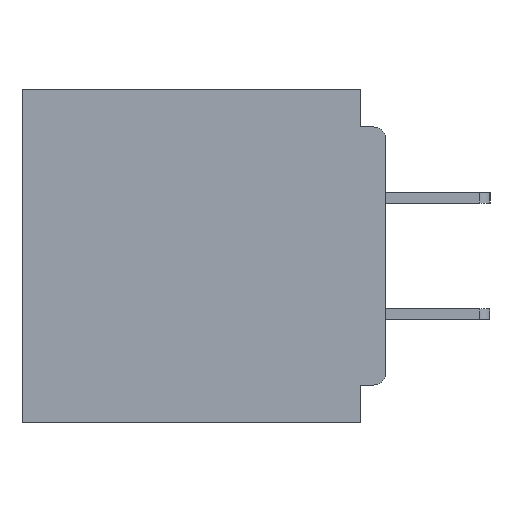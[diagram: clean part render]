
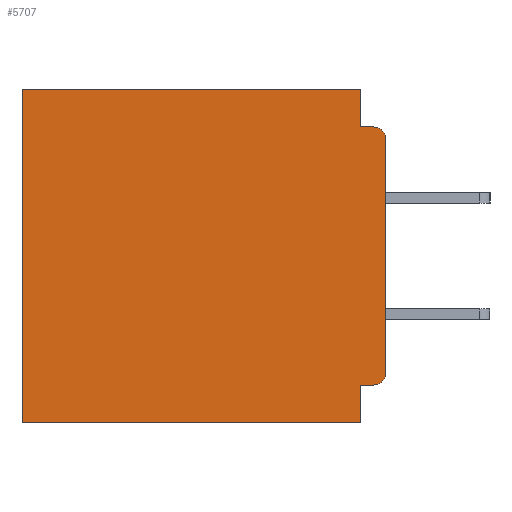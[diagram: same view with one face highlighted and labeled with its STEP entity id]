
A CAD part, left-side view. The second image highlights one B-rep face of the part: STEP entity #5707.
In plain terms, the highlighted planar face has unit normal (-1, 0, 0).
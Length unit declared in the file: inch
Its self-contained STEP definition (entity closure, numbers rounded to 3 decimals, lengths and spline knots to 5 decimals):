
#2640 = CARTESIAN_POINT ( 'NONE',  ( 0.3, 0.031, -0.045 ) ) ;
#3338 = CARTESIAN_POINT ( 'NONE',  ( 0.3, 0.031, -0.355 ) ) ;
#3873 = VECTOR ( 'NONE', #16512, 39.37008 ) ;
#4397 = EDGE_CURVE ( 'NONE', #32176, #6523, #39195, .T. ) ;
#4550 = EDGE_CURVE ( 'NONE', #6523, #17358, #5395, .T. ) ;
#4761 = CARTESIAN_POINT ( 'NONE',  ( 0.3, 0., -0.06 ) ) ;
#4972 = EDGE_LOOP ( 'NONE', ( #5251, #22607, #36116, #38105, #28368, #12753, #35700, #60709, #61711, #25849 ) ) ;
#5251 = ORIENTED_EDGE ( 'NONE', *, *, #47994, .F. ) ;
#5395 = LINE ( 'NONE', #31305, #3873 ) ;
#5631 = CIRCLE ( 'NONE', #12392, 0.015 ) ;
#5706 = EDGE_CURVE ( 'NONE', #32176, #54962, #39880, .T. ) ;
#5707 = ADVANCED_FACE ( 'NONE', ( #54378 ), #25562, .F. ) ;
#6001 = DIRECTION ( 'NONE',  ( -1., 0., 0. ) ) ;
#6523 = VERTEX_POINT ( 'NONE', #3338 ) ;
#7108 = LINE ( 'NONE', #30990, #31738 ) ;
#8155 = CARTESIAN_POINT ( 'NONE',  ( 0.3, 0., -0.34 ) ) ;
#8298 = CARTESIAN_POINT ( 'NONE',  ( 0.3, 0.437, -0.4 ) ) ;
#8431 = LINE ( 'NONE', #8298, #19957 ) ;
#9497 = CARTESIAN_POINT ( 'NONE',  ( 0.3, 0., -0.4 ) ) ;
#10766 = CARTESIAN_POINT ( 'NONE',  ( 0.3, 0.015, -0.355 ) ) ;
#10851 = VECTOR ( 'NONE', #26500, 39.37008 ) ;
#10919 = DIRECTION ( 'NONE',  ( 1., 0., 0. ) ) ;
#11439 = AXIS2_PLACEMENT_3D ( 'NONE', #35404, #6001, #40308 ) ;
#12392 = AXIS2_PLACEMENT_3D ( 'NONE', #43758, #14448, #48666 ) ;
#12753 = ORIENTED_EDGE ( 'NONE', *, *, #14471, .T. ) ;
#13203 = CARTESIAN_POINT ( 'NONE',  ( 0.3, 0., 0. ) ) ;
#13997 = CARTESIAN_POINT ( 'NONE',  ( 0.3, 0.437, -0.4 ) ) ;
#14448 = DIRECTION ( 'NONE',  ( -1., 0., 0. ) ) ;
#14471 = EDGE_CURVE ( 'NONE', #35315, #16813, #8431, .T. ) ;
#15427 = DIRECTION ( 'NONE',  ( 0., 1., 0. ) ) ;
#16512 = DIRECTION ( 'NONE',  ( 0., 0., -1. ) ) ;
#16813 = VERTEX_POINT ( 'NONE', #13997 ) ;
#17358 = VERTEX_POINT ( 'NONE', #57992 ) ;
#18377 = CARTESIAN_POINT ( 'NONE',  ( 0.3, 0., -0.4 ) ) ;
#19957 = VECTOR ( 'NONE', #37678, 39.37008 ) ;
#20743 = CARTESIAN_POINT ( 'NONE',  ( 0.3, 0.015, -0.045 ) ) ;
#22418 = LINE ( 'NONE', #55731, #10851 ) ;
#22607 = ORIENTED_EDGE ( 'NONE', *, *, #32516, .T. ) ;
#23160 = VECTOR ( 'NONE', #57064, 39.37008 ) ;
#24619 = AXIS2_PLACEMENT_3D ( 'NONE', #40106, #10919, #45216 ) ;
#25562 = PLANE ( 'NONE',  #24619 ) ;
#25849 = ORIENTED_EDGE ( 'NONE', *, *, #5706, .T. ) ;
#26191 = VECTOR ( 'NONE', #15427, 39.37008 ) ;
#26319 = EDGE_CURVE ( 'NONE', #17358, #16813, #45358, .T. ) ;
#26500 = DIRECTION ( 'NONE',  ( 0., 0., -1. ) ) ;
#28368 = ORIENTED_EDGE ( 'NONE', *, *, #37633, .T. ) ;
#29268 = DIRECTION ( 'NONE',  ( 0., 1., 0. ) ) ;
#30990 = CARTESIAN_POINT ( 'NONE',  ( 0.3, 0., -0.045 ) ) ;
#31305 = CARTESIAN_POINT ( 'NONE',  ( 0.3, 0.031, -0.4 ) ) ;
#31358 = VECTOR ( 'NONE', #47911, 39.37008 ) ;
#31667 = VERTEX_POINT ( 'NONE', #55801 ) ;
#31738 = VECTOR ( 'NONE', #35857, 39.37008 ) ;
#32176 = VERTEX_POINT ( 'NONE', #10766 ) ;
#32296 = VERTEX_POINT ( 'NONE', #2640 ) ;
#32516 = EDGE_CURVE ( 'NONE', #44482, #39981, #5631, .T. ) ;
#35315 = VERTEX_POINT ( 'NONE', #58834 ) ;
#35404 = CARTESIAN_POINT ( 'NONE',  ( 0.3, 0.015, -0.34 ) ) ;
#35700 = ORIENTED_EDGE ( 'NONE', *, *, #26319, .F. ) ;
#35857 = DIRECTION ( 'NONE',  ( 0., -1., 0. ) ) ;
#36116 = ORIENTED_EDGE ( 'NONE', *, *, #50802, .F. ) ;
#37633 = EDGE_CURVE ( 'NONE', #31667, #35315, #62126, .T. ) ;
#37678 = DIRECTION ( 'NONE',  ( 0., 0., -1. ) ) ;
#38103 = EDGE_CURVE ( 'NONE', #31667, #32296, #22418, .T. ) ;
#38105 = ORIENTED_EDGE ( 'NONE', *, *, #38103, .F. ) ;
#39195 = LINE ( 'NONE', #39841, #26191 ) ;
#39841 = CARTESIAN_POINT ( 'NONE',  ( 0.3, 0., -0.355 ) ) ;
#39880 = CIRCLE ( 'NONE', #11439, 0.015 ) ;
#39981 = VERTEX_POINT ( 'NONE', #20743 ) ;
#40106 = CARTESIAN_POINT ( 'NONE',  ( 0.3, 0., -0.4 ) ) ;
#40308 = DIRECTION ( 'NONE',  ( 0., 0., -1. ) ) ;
#43758 = CARTESIAN_POINT ( 'NONE',  ( 0.3, 0.015, -0.06 ) ) ;
#44318 = LINE ( 'NONE', #18377, #31358 ) ;
#44482 = VERTEX_POINT ( 'NONE', #4761 ) ;
#45216 = DIRECTION ( 'NONE',  ( 0., 0., -1. ) ) ;
#45358 = LINE ( 'NONE', #9497, #56820 ) ;
#47911 = DIRECTION ( 'NONE',  ( 0., 0., -1. ) ) ;
#47994 = EDGE_CURVE ( 'NONE', #44482, #54962, #44318, .T. ) ;
#48666 = DIRECTION ( 'NONE',  ( 0., 0., -1. ) ) ;
#50802 = EDGE_CURVE ( 'NONE', #32296, #39981, #7108, .T. ) ;
#54378 = FACE_OUTER_BOUND ( 'NONE', #4972, .T. ) ;
#54962 = VERTEX_POINT ( 'NONE', #8155 ) ;
#55731 = CARTESIAN_POINT ( 'NONE',  ( 0.3, 0.031, 0. ) ) ;
#55801 = CARTESIAN_POINT ( 'NONE',  ( 0.3, 0.031, 0. ) ) ;
#56820 = VECTOR ( 'NONE', #29268, 39.37008 ) ;
#57064 = DIRECTION ( 'NONE',  ( 0., 1., 0. ) ) ;
#57992 = CARTESIAN_POINT ( 'NONE',  ( 0.3, 0.031, -0.4 ) ) ;
#58834 = CARTESIAN_POINT ( 'NONE',  ( 0.3, 0.437, 0. ) ) ;
#60709 = ORIENTED_EDGE ( 'NONE', *, *, #4550, .F. ) ;
#61711 = ORIENTED_EDGE ( 'NONE', *, *, #4397, .F. ) ;
#62126 = LINE ( 'NONE', #13203, #23160 ) ;
